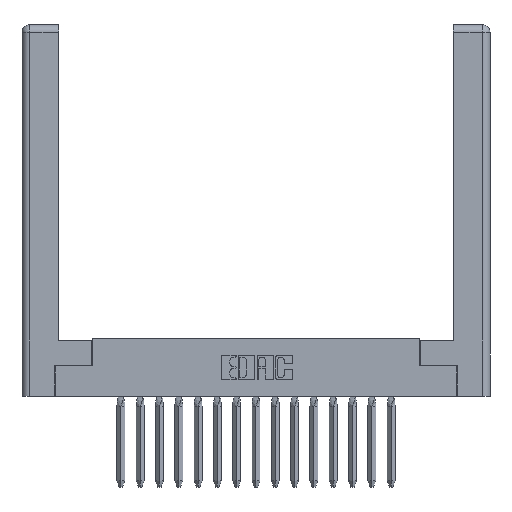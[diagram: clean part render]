
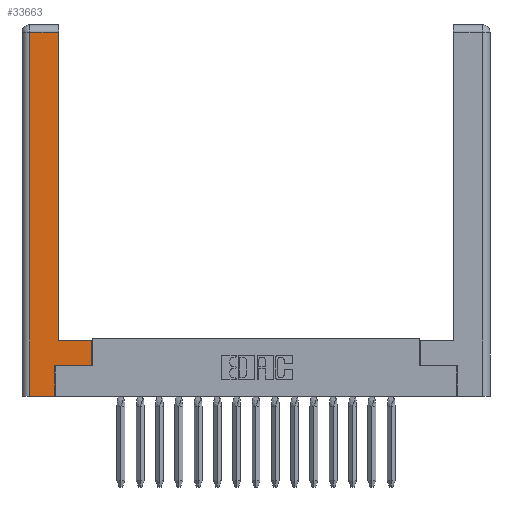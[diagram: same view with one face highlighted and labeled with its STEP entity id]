
A CAD part, top view. The second image highlights one B-rep face of the part: STEP entity #33663.
In plain terms, the highlighted planar face has unit normal (0, 0, 1).
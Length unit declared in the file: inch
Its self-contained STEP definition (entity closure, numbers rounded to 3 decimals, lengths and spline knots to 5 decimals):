
#268 = CARTESIAN_POINT ( 'NONE',  ( 0.0615, 2.94, 0. ) ) ;
#644 = LINE ( 'NONE', #26943, #20596 ) ;
#891 = VERTEX_POINT ( 'NONE', #2038 ) ;
#1905 = VECTOR ( 'NONE', #3534, 39.37008 ) ;
#2038 = CARTESIAN_POINT ( 'NONE',  ( 0.295, 0.45, 0. ) ) ;
#2477 = VERTEX_POINT ( 'NONE', #19270 ) ;
#2643 = LINE ( 'NONE', #15517, #22147 ) ;
#2995 = VERTEX_POINT ( 'NONE', #4462 ) ;
#3534 = DIRECTION ( 'NONE',  ( -1., 0., 0. ) ) ;
#3636 = DIRECTION ( 'NONE',  ( 0., -1., 0. ) ) ;
#4315 = EDGE_CURVE ( 'NONE', #891, #13645, #644, .T. ) ;
#4462 = CARTESIAN_POINT ( 'NONE',  ( 0.565, 0.245, 0. ) ) ;
#5775 = CARTESIAN_POINT ( 'NONE',  ( 0., 0., 0. ) ) ;
#5840 = EDGE_CURVE ( 'NONE', #2995, #2477, #2643, .T. ) ;
#6120 = VERTEX_POINT ( 'NONE', #14583 ) ;
#6166 = ORIENTED_EDGE ( 'NONE', *, *, #23948, .T. ) ;
#6604 = CARTESIAN_POINT ( 'NONE',  ( 0.265, 0.245, 0. ) ) ;
#6911 = CARTESIAN_POINT ( 'NONE',  ( 0.295, 2.94, 0. ) ) ;
#8433 = PLANE ( 'NONE',  #13546 ) ;
#9956 = DIRECTION ( 'NONE',  ( 1., 0., 0. ) ) ;
#10515 = EDGE_CURVE ( 'NONE', #32788, #6120, #22919, .T. ) ;
#10969 = DIRECTION ( 'NONE',  ( 1., 0., 0. ) ) ;
#12548 = VECTOR ( 'NONE', #9956, 39.37008 ) ;
#13447 = DIRECTION ( 'NONE',  ( 0., 0., -1. ) ) ;
#13546 = AXIS2_PLACEMENT_3D ( 'NONE', #5775, #13447, #26974 ) ;
#13645 = VERTEX_POINT ( 'NONE', #6911 ) ;
#13994 = CARTESIAN_POINT ( 'NONE',  ( 0.295, 0.45, 0. ) ) ;
#14000 = CARTESIAN_POINT ( 'NONE',  ( 0.0615, 0., 0. ) ) ;
#14583 = CARTESIAN_POINT ( 'NONE',  ( 0.265, 0., 0. ) ) ;
#15265 = ORIENTED_EDGE ( 'NONE', *, *, #24583, .T. ) ;
#15517 = CARTESIAN_POINT ( 'NONE',  ( 0.565, 0.45, 0. ) ) ;
#15985 = VECTOR ( 'NONE', #22499, 39.37008 ) ;
#16040 = LINE ( 'NONE', #29684, #32903 ) ;
#16797 = ORIENTED_EDGE ( 'NONE', *, *, #23421, .T. ) ;
#17283 = VERTEX_POINT ( 'NONE', #21976 ) ;
#18244 = DIRECTION ( 'NONE',  ( -1., 0., 0. ) ) ;
#19270 = CARTESIAN_POINT ( 'NONE',  ( 0.565, 0.45, 0. ) ) ;
#19958 = LINE ( 'NONE', #27179, #29868 ) ;
#20596 = VECTOR ( 'NONE', #21515, 39.37008 ) ;
#21052 = ORIENTED_EDGE ( 'NONE', *, *, #10515, .T. ) ;
#21515 = DIRECTION ( 'NONE',  ( 0., 1., 0. ) ) ;
#21976 = CARTESIAN_POINT ( 'NONE',  ( 0.265, 0.245, 0. ) ) ;
#22147 = VECTOR ( 'NONE', #26282, 39.37008 ) ;
#22499 = DIRECTION ( 'NONE',  ( 0., 1., 0. ) ) ;
#22919 = LINE ( 'NONE', #28385, #12548 ) ;
#23421 = EDGE_CURVE ( 'NONE', #2477, #891, #27603, .T. ) ;
#23539 = EDGE_CURVE ( 'NONE', #26312, #32788, #16040, .T. ) ;
#23948 = EDGE_CURVE ( 'NONE', #13645, #26312, #24013, .T. ) ;
#24013 = LINE ( 'NONE', #31700, #30116 ) ;
#24583 = EDGE_CURVE ( 'NONE', #17283, #2995, #19958, .T. ) ;
#24988 = FACE_OUTER_BOUND ( 'NONE', #25128, .T. ) ;
#25128 = EDGE_LOOP ( 'NONE', ( #26019, #6166, #31731, #21052, #29190, #15265, #28103, #16797 ) ) ;
#26019 = ORIENTED_EDGE ( 'NONE', *, *, #4315, .T. ) ;
#26282 = DIRECTION ( 'NONE',  ( 0., 1., 0. ) ) ;
#26312 = VERTEX_POINT ( 'NONE', #268 ) ;
#26943 = CARTESIAN_POINT ( 'NONE',  ( 0.295, 3., 0. ) ) ;
#26974 = DIRECTION ( 'NONE',  ( -1., 0., 0. ) ) ;
#27179 = CARTESIAN_POINT ( 'NONE',  ( 0.565, 0.245, 0. ) ) ;
#27603 = LINE ( 'NONE', #13994, #1905 ) ;
#28103 = ORIENTED_EDGE ( 'NONE', *, *, #5840, .T. ) ;
#28385 = CARTESIAN_POINT ( 'NONE',  ( 0.265, 0., 0. ) ) ;
#29190 = ORIENTED_EDGE ( 'NONE', *, *, #32346, .T. ) ;
#29684 = CARTESIAN_POINT ( 'NONE',  ( 0.0615, 0., 0. ) ) ;
#29868 = VECTOR ( 'NONE', #10969, 39.37008 ) ;
#30116 = VECTOR ( 'NONE', #18244, 39.37008 ) ;
#31700 = CARTESIAN_POINT ( 'NONE',  ( 0.0615, 2.94, 0. ) ) ;
#31731 = ORIENTED_EDGE ( 'NONE', *, *, #23539, .T. ) ;
#32346 = EDGE_CURVE ( 'NONE', #6120, #17283, #32853, .T. ) ;
#32788 = VERTEX_POINT ( 'NONE', #14000 ) ;
#32853 = LINE ( 'NONE', #6604, #15985 ) ;
#32903 = VECTOR ( 'NONE', #3636, 39.37008 ) ;
#33663 = ADVANCED_FACE ( 'NONE', ( #24988 ), #8433, .F. ) ;
